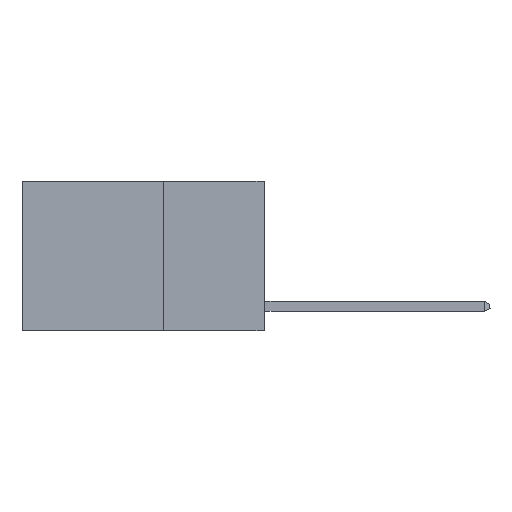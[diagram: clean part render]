
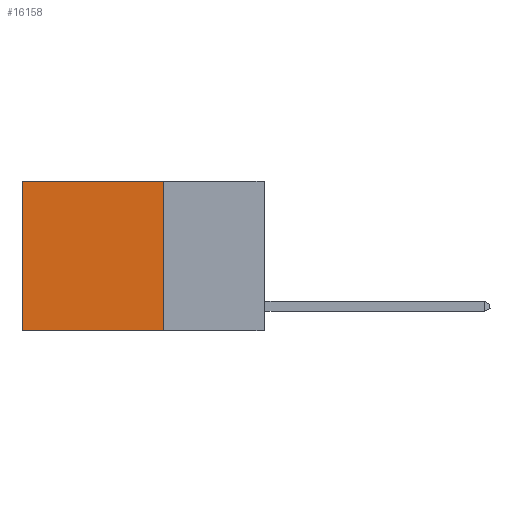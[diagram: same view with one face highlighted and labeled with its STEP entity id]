
A CAD part, left-side view. The second image highlights one B-rep face of the part: STEP entity #16158.
In plain terms, the highlighted planar face has unit normal (-1, 0, 0).
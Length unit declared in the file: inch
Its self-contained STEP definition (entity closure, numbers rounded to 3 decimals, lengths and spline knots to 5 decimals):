
#780 = CARTESIAN_POINT ( 'NONE',  ( 0.2625, 0.25, 0. ) ) ;
#2003 = VECTOR ( 'NONE', #18187, 39.37008 ) ;
#2420 = VERTEX_POINT ( 'NONE', #780 ) ;
#3370 = VERTEX_POINT ( 'NONE', #22416 ) ;
#3427 = CARTESIAN_POINT ( 'NONE',  ( 0.2625, 0.6, -0.37 ) ) ;
#3850 = ORIENTED_EDGE ( 'NONE', *, *, #17319, .F. ) ;
#4059 = VERTEX_POINT ( 'NONE', #3427 ) ;
#4494 = PLANE ( 'NONE',  #13336 ) ;
#4719 = FACE_OUTER_BOUND ( 'NONE', #13664, .T. ) ;
#5183 = EDGE_CURVE ( 'NONE', #2420, #3370, #16629, .T. ) ;
#5262 = VECTOR ( 'NONE', #20564, 39.37008 ) ;
#8605 = DIRECTION ( 'NONE',  ( 1., 0., 0. ) ) ;
#8939 = EDGE_CURVE ( 'NONE', #21895, #4059, #22885, .T. ) ;
#9178 = ORIENTED_EDGE ( 'NONE', *, *, #8939, .F. ) ;
#9684 = CARTESIAN_POINT ( 'NONE',  ( 0.2625, 0.25, 0. ) ) ;
#12027 = LINE ( 'NONE', #19590, #2003 ) ;
#13336 = AXIS2_PLACEMENT_3D ( 'NONE', #20199, #8605, #23972 ) ;
#13664 = EDGE_LOOP ( 'NONE', ( #23957, #9178, #3850, #16456 ) ) ;
#13884 = DIRECTION ( 'NONE',  ( 0., 1., 0. ) ) ;
#15291 = CARTESIAN_POINT ( 'NONE',  ( 0.2625, 0.25, -0.37 ) ) ;
#16158 = ADVANCED_FACE ( 'NONE', ( #4719 ), #4494, .F. ) ;
#16456 = ORIENTED_EDGE ( 'NONE', *, *, #5183, .T. ) ;
#16629 = LINE ( 'NONE', #18786, #5262 ) ;
#17319 = EDGE_CURVE ( 'NONE', #2420, #21895, #19508, .T. ) ;
#17592 = DIRECTION ( 'NONE',  ( 0., 0., -1. ) ) ;
#18162 = VECTOR ( 'NONE', #17592, 39.37008 ) ;
#18187 = DIRECTION ( 'NONE',  ( 0., 0., -1. ) ) ;
#18786 = CARTESIAN_POINT ( 'NONE',  ( 0.2625, 0.25, 0. ) ) ;
#19508 = LINE ( 'NONE', #9684, #18162 ) ;
#19590 = CARTESIAN_POINT ( 'NONE',  ( 0.2625, 0.6, 0. ) ) ;
#20199 = CARTESIAN_POINT ( 'NONE',  ( 0.2625, 0.25, 0. ) ) ;
#20564 = DIRECTION ( 'NONE',  ( 0., 1., 0. ) ) ;
#20573 = EDGE_CURVE ( 'NONE', #3370, #4059, #12027, .T. ) ;
#21895 = VERTEX_POINT ( 'NONE', #22628 ) ;
#22416 = CARTESIAN_POINT ( 'NONE',  ( 0.2625, 0.6, 0. ) ) ;
#22628 = CARTESIAN_POINT ( 'NONE',  ( 0.2625, 0.25, -0.37 ) ) ;
#22885 = LINE ( 'NONE', #15291, #24118 ) ;
#23957 = ORIENTED_EDGE ( 'NONE', *, *, #20573, .T. ) ;
#23972 = DIRECTION ( 'NONE',  ( 0., 0., -1. ) ) ;
#24118 = VECTOR ( 'NONE', #13884, 39.37008 ) ;
